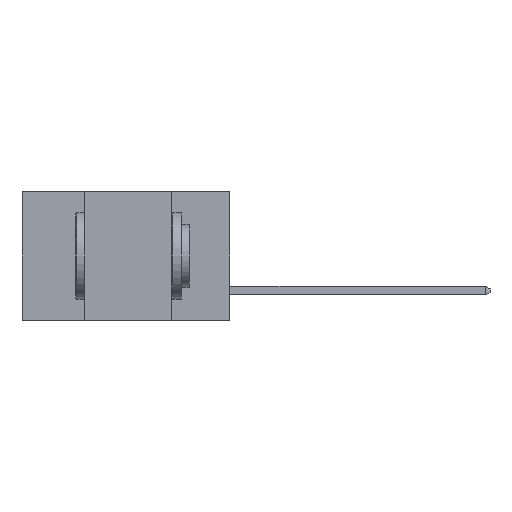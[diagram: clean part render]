
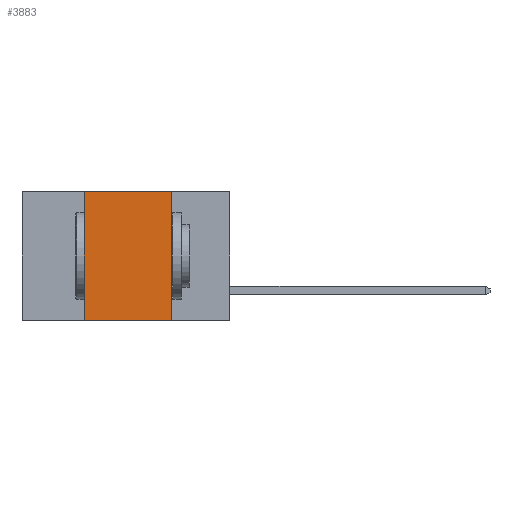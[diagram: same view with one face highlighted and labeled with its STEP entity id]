
A CAD part, left-side view. The second image highlights one B-rep face of the part: STEP entity #3883.
In plain terms, the highlighted planar face has unit normal (-1, 0, 0).
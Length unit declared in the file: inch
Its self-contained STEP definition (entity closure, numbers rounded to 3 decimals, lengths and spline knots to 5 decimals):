
#829 = DIRECTION ( 'NONE',  ( 0., -1., 0. ) ) ;
#2374 = CARTESIAN_POINT ( 'NONE',  ( 0., 0.17, 0. ) ) ;
#2442 = LINE ( 'NONE', #10179, #13805 ) ;
#2542 = ORIENTED_EDGE ( 'NONE', *, *, #6213, .F. ) ;
#2569 = VERTEX_POINT ( 'NONE', #4646 ) ;
#2791 = VECTOR ( 'NONE', #10526, 39.37008 ) ;
#2828 = EDGE_CURVE ( 'NONE', #2569, #13625, #13141, .T. ) ;
#2946 = DIRECTION ( 'NONE',  ( 1., 0., 0. ) ) ;
#3302 = DIRECTION ( 'NONE',  ( 0., -1., 0. ) ) ;
#3883 = ADVANCED_FACE ( 'NONE', ( #6422 ), #10776, .F. ) ;
#4322 = VECTOR ( 'NONE', #829, 39.37008 ) ;
#4472 = LINE ( 'NONE', #4940, #2791 ) ;
#4646 = CARTESIAN_POINT ( 'NONE',  ( 0., 0.42, 0. ) ) ;
#4677 = DIRECTION ( 'NONE',  ( 0., 0., -1. ) ) ;
#4940 = CARTESIAN_POINT ( 'NONE',  ( 0., 0.42, -0.37 ) ) ;
#5248 = EDGE_CURVE ( 'NONE', #13625, #12865, #2442, .T. ) ;
#5287 = CARTESIAN_POINT ( 'NONE',  ( 0., 0.6, 0. ) ) ;
#5817 = ORIENTED_EDGE ( 'NONE', *, *, #2828, .F. ) ;
#6213 = EDGE_CURVE ( 'NONE', #8813, #2569, #4472, .T. ) ;
#6422 = FACE_OUTER_BOUND ( 'NONE', #13977, .T. ) ;
#7365 = DIRECTION ( 'NONE',  ( 0., 0., -1. ) ) ;
#7431 = CARTESIAN_POINT ( 'NONE',  ( 0., 0.6, -0.37 ) ) ;
#7498 = ORIENTED_EDGE ( 'NONE', *, *, #9551, .T. ) ;
#8813 = VERTEX_POINT ( 'NONE', #9409 ) ;
#9409 = CARTESIAN_POINT ( 'NONE',  ( 0., 0.42, -0.37 ) ) ;
#9551 = EDGE_CURVE ( 'NONE', #8813, #12865, #10350, .T. ) ;
#9777 = CARTESIAN_POINT ( 'NONE',  ( 0., 0.17, -0.37 ) ) ;
#10179 = CARTESIAN_POINT ( 'NONE',  ( 0., 0.17, -0.37 ) ) ;
#10350 = LINE ( 'NONE', #7431, #4322 ) ;
#10526 = DIRECTION ( 'NONE',  ( 0., 0., 1. ) ) ;
#10699 = AXIS2_PLACEMENT_3D ( 'NONE', #5287, #2946, #7365 ) ;
#10776 = PLANE ( 'NONE',  #10699 ) ;
#10897 = VECTOR ( 'NONE', #3302, 39.37008 ) ;
#12865 = VERTEX_POINT ( 'NONE', #9777 ) ;
#13141 = LINE ( 'NONE', #13211, #10897 ) ;
#13211 = CARTESIAN_POINT ( 'NONE',  ( 0., 0.6, 0. ) ) ;
#13625 = VERTEX_POINT ( 'NONE', #2374 ) ;
#13805 = VECTOR ( 'NONE', #4677, 39.37008 ) ;
#13934 = ORIENTED_EDGE ( 'NONE', *, *, #5248, .F. ) ;
#13977 = EDGE_LOOP ( 'NONE', ( #13934, #5817, #2542, #7498 ) ) ;
